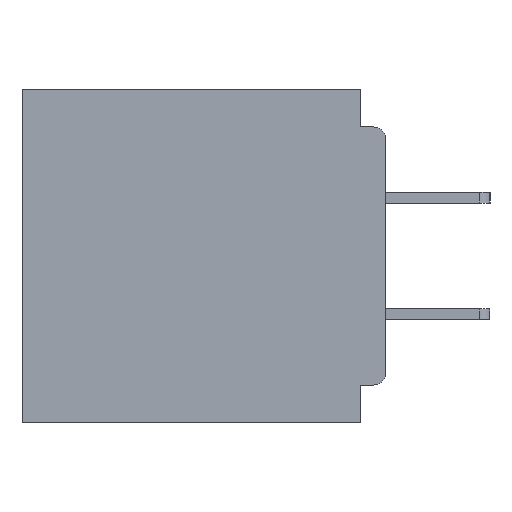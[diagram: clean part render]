
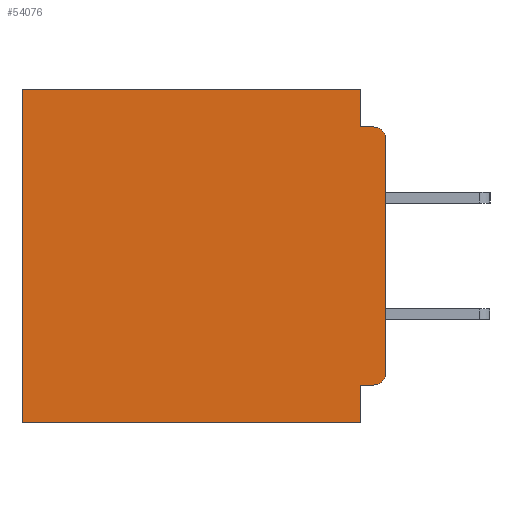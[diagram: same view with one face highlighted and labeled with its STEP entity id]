
A CAD part, left-side view. The second image highlights one B-rep face of the part: STEP entity #54076.
In plain terms, the highlighted planar face has unit normal (-1, 0, 0).
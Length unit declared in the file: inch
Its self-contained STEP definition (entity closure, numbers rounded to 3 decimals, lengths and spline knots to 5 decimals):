
#358 = CARTESIAN_POINT ( 'NONE',  ( 0.3, 0.437, -0.4 ) ) ;
#1024 = VECTOR ( 'NONE', #17342, 39.37008 ) ;
#1314 = EDGE_CURVE ( 'NONE', #24404, #27177, #16682, .T. ) ;
#2405 = VERTEX_POINT ( 'NONE', #48524 ) ;
#2436 = EDGE_CURVE ( 'NONE', #51431, #45470, #5665, .T. ) ;
#4266 = DIRECTION ( 'NONE',  ( -1., 0., 0. ) ) ;
#4345 = VECTOR ( 'NONE', #13695, 39.37008 ) ;
#5291 = CARTESIAN_POINT ( 'NONE',  ( 0.3, 0.437, 0. ) ) ;
#5413 = EDGE_CURVE ( 'NONE', #2405, #45470, #36693, .T. ) ;
#5437 = LINE ( 'NONE', #6022, #26757 ) ;
#5665 = LINE ( 'NONE', #9085, #4345 ) ;
#6022 = CARTESIAN_POINT ( 'NONE',  ( 0.3, 0., -0.045 ) ) ;
#7243 = ORIENTED_EDGE ( 'NONE', *, *, #38849, .F. ) ;
#7346 = ORIENTED_EDGE ( 'NONE', *, *, #1314, .F. ) ;
#8143 = ORIENTED_EDGE ( 'NONE', *, *, #2436, .F. ) ;
#9085 = CARTESIAN_POINT ( 'NONE',  ( 0.3, 0., -0.4 ) ) ;
#9261 = CARTESIAN_POINT ( 'NONE',  ( 0.3, 0.031, 0. ) ) ;
#10245 = VECTOR ( 'NONE', #43075, 39.37008 ) ;
#10485 = EDGE_CURVE ( 'NONE', #34295, #49514, #52825, .T. ) ;
#10523 = EDGE_LOOP ( 'NONE', ( #8143, #54487, #7243, #51118, #38152, #39258, #49623, #7346, #18686, #28014 ) ) ;
#11046 = LINE ( 'NONE', #42662, #1024 ) ;
#11300 = DIRECTION ( 'NONE',  ( 0., 1., 0. ) ) ;
#11418 = CARTESIAN_POINT ( 'NONE',  ( 0.3, 0.031, 0. ) ) ;
#12547 = CARTESIAN_POINT ( 'NONE',  ( 0.3, 0.015, -0.045 ) ) ;
#13586 = DIRECTION ( 'NONE',  ( 0., 0., -1. ) ) ;
#13695 = DIRECTION ( 'NONE',  ( 0., 0., -1. ) ) ;
#14276 = LINE ( 'NONE', #17764, #10245 ) ;
#15464 = CARTESIAN_POINT ( 'NONE',  ( 0.3, 0.031, -0.045 ) ) ;
#15660 = FACE_OUTER_BOUND ( 'NONE', #10523, .T. ) ;
#16682 = LINE ( 'NONE', #20076, #37872 ) ;
#17342 = DIRECTION ( 'NONE',  ( 0., 1., 0. ) ) ;
#17764 = CARTESIAN_POINT ( 'NONE',  ( 0.3, 0., 0. ) ) ;
#17857 = VECTOR ( 'NONE', #13586, 39.37008 ) ;
#18411 = CIRCLE ( 'NONE', #21744, 0.015 ) ;
#18686 = ORIENTED_EDGE ( 'NONE', *, *, #35042, .F. ) ;
#18956 = CARTESIAN_POINT ( 'NONE',  ( 0.3, 0., -0.34 ) ) ;
#20075 = CARTESIAN_POINT ( 'NONE',  ( 0.3, 0.031, -0.355 ) ) ;
#20076 = CARTESIAN_POINT ( 'NONE',  ( 0.3, 0.031, -0.4 ) ) ;
#21744 = AXIS2_PLACEMENT_3D ( 'NONE', #29749, #4266, #34036 ) ;
#22287 = CARTESIAN_POINT ( 'NONE',  ( 0.3, 0.015, -0.34 ) ) ;
#22335 = VERTEX_POINT ( 'NONE', #5291 ) ;
#22673 = CARTESIAN_POINT ( 'NONE',  ( 0.3, 0.437, -0.4 ) ) ;
#23028 = DIRECTION ( 'NONE',  ( 0., -1., 0. ) ) ;
#23385 = EDGE_CURVE ( 'NONE', #34295, #22335, #14276, .T. ) ;
#23652 = CARTESIAN_POINT ( 'NONE',  ( 0.3, 0., -0.4 ) ) ;
#23954 = CARTESIAN_POINT ( 'NONE',  ( 0.3, 0., -0.4 ) ) ;
#24136 = EDGE_CURVE ( 'NONE', #22335, #50930, #50565, .T. ) ;
#24370 = EDGE_CURVE ( 'NONE', #27177, #50930, #49885, .T. ) ;
#24404 = VERTEX_POINT ( 'NONE', #20075 ) ;
#26507 = DIRECTION ( 'NONE',  ( 0., 0., -1. ) ) ;
#26757 = VECTOR ( 'NONE', #23028, 39.37008 ) ;
#27177 = VERTEX_POINT ( 'NONE', #36275 ) ;
#27852 = DIRECTION ( 'NONE',  ( 0., 0., -1. ) ) ;
#28014 = ORIENTED_EDGE ( 'NONE', *, *, #5413, .T. ) ;
#29749 = CARTESIAN_POINT ( 'NONE',  ( 0.3, 0.015, -0.06 ) ) ;
#29991 = DIRECTION ( 'NONE',  ( 0., 0., -1. ) ) ;
#31153 = DIRECTION ( 'NONE',  ( 0., 0., -1. ) ) ;
#32872 = AXIS2_PLACEMENT_3D ( 'NONE', #23652, #53126, #27852 ) ;
#34036 = DIRECTION ( 'NONE',  ( 0., 0., -1. ) ) ;
#34295 = VERTEX_POINT ( 'NONE', #11418 ) ;
#35042 = EDGE_CURVE ( 'NONE', #2405, #24404, #11046, .T. ) ;
#36242 = VERTEX_POINT ( 'NONE', #12547 ) ;
#36275 = CARTESIAN_POINT ( 'NONE',  ( 0.3, 0.031, -0.4 ) ) ;
#36693 = CIRCLE ( 'NONE', #41197, 0.015 ) ;
#37872 = VECTOR ( 'NONE', #29991, 39.37008 ) ;
#38049 = VECTOR ( 'NONE', #31153, 39.37008 ) ;
#38152 = ORIENTED_EDGE ( 'NONE', *, *, #23385, .T. ) ;
#38681 = VECTOR ( 'NONE', #11300, 39.37008 ) ;
#38849 = EDGE_CURVE ( 'NONE', #49514, #36242, #5437, .T. ) ;
#39258 = ORIENTED_EDGE ( 'NONE', *, *, #24136, .T. ) ;
#40471 = PLANE ( 'NONE',  #32872 ) ;
#41197 = AXIS2_PLACEMENT_3D ( 'NONE', #22287, #51766, #26507 ) ;
#42561 = EDGE_CURVE ( 'NONE', #51431, #36242, #18411, .T. ) ;
#42662 = CARTESIAN_POINT ( 'NONE',  ( 0.3, 0., -0.355 ) ) ;
#43075 = DIRECTION ( 'NONE',  ( 0., 1., 0. ) ) ;
#45470 = VERTEX_POINT ( 'NONE', #18956 ) ;
#48524 = CARTESIAN_POINT ( 'NONE',  ( 0.3, 0.015, -0.355 ) ) ;
#49416 = CARTESIAN_POINT ( 'NONE',  ( 0.3, 0., -0.06 ) ) ;
#49514 = VERTEX_POINT ( 'NONE', #15464 ) ;
#49623 = ORIENTED_EDGE ( 'NONE', *, *, #24370, .F. ) ;
#49885 = LINE ( 'NONE', #23954, #38681 ) ;
#50565 = LINE ( 'NONE', #22673, #38049 ) ;
#50930 = VERTEX_POINT ( 'NONE', #358 ) ;
#51118 = ORIENTED_EDGE ( 'NONE', *, *, #10485, .F. ) ;
#51431 = VERTEX_POINT ( 'NONE', #49416 ) ;
#51766 = DIRECTION ( 'NONE',  ( -1., 0., 0. ) ) ;
#52825 = LINE ( 'NONE', #9261, #17857 ) ;
#53126 = DIRECTION ( 'NONE',  ( 1., 0., 0. ) ) ;
#54076 = ADVANCED_FACE ( 'NONE', ( #15660 ), #40471, .F. ) ;
#54487 = ORIENTED_EDGE ( 'NONE', *, *, #42561, .T. ) ;
